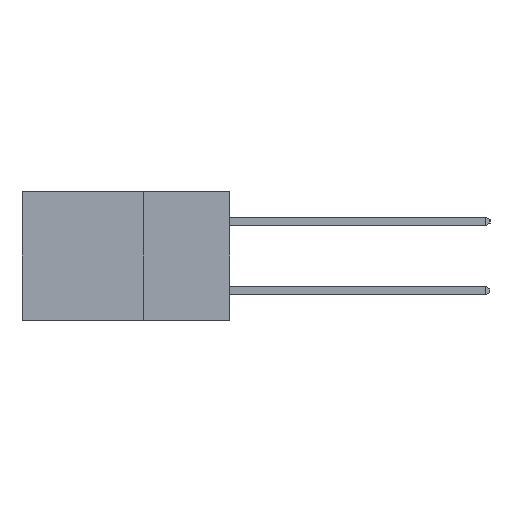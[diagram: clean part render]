
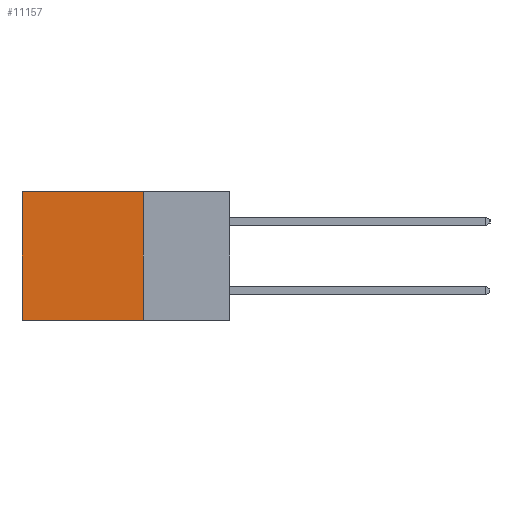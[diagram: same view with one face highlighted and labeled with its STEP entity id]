
A CAD part, left-side view. The second image highlights one B-rep face of the part: STEP entity #11157.
In plain terms, the highlighted planar face has unit normal (-1, 0, 0).
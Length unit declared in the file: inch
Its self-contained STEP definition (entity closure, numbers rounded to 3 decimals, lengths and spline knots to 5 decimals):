
#114 = CARTESIAN_POINT ( 'NONE',  ( 0.298, 0.6, 0. ) ) ;
#216 = VECTOR ( 'NONE', #2900, 39.37008 ) ;
#567 = VECTOR ( 'NONE', #4350, 39.37008 ) ;
#844 = ORIENTED_EDGE ( 'NONE', *, *, #13012, .T. ) ;
#1323 = LINE ( 'NONE', #11193, #3573 ) ;
#1818 = DIRECTION ( 'NONE',  ( 0., 0., -1. ) ) ;
#1837 = DIRECTION ( 'NONE',  ( 1., 0., 0. ) ) ;
#1908 = PLANE ( 'NONE',  #3236 ) ;
#1910 = ORIENTED_EDGE ( 'NONE', *, *, #11044, .T. ) ;
#1998 = VERTEX_POINT ( 'NONE', #114 ) ;
#2043 = CARTESIAN_POINT ( 'NONE',  ( 0.298, 0.25, 0. ) ) ;
#2697 = EDGE_LOOP ( 'NONE', ( #844, #6848, #4448, #1910 ) ) ;
#2900 = DIRECTION ( 'NONE',  ( 0., 1., 0. ) ) ;
#2950 = CARTESIAN_POINT ( 'NONE',  ( 0.298, 0.25, 0. ) ) ;
#3070 = CARTESIAN_POINT ( 'NONE',  ( 0.298, 0.6, 0. ) ) ;
#3236 = AXIS2_PLACEMENT_3D ( 'NONE', #2043, #1837, #1818 ) ;
#3573 = VECTOR ( 'NONE', #6476, 39.37008 ) ;
#4350 = DIRECTION ( 'NONE',  ( 0., 0., -1. ) ) ;
#4448 = ORIENTED_EDGE ( 'NONE', *, *, #4717, .F. ) ;
#4514 = VERTEX_POINT ( 'NONE', #5156 ) ;
#4717 = EDGE_CURVE ( 'NONE', #9483, #9726, #15726, .T. ) ;
#5156 = CARTESIAN_POINT ( 'NONE',  ( 0.298, 0.6, -0.37 ) ) ;
#6476 = DIRECTION ( 'NONE',  ( 0., 1., 0. ) ) ;
#6848 = ORIENTED_EDGE ( 'NONE', *, *, #14731, .F. ) ;
#8232 = FACE_OUTER_BOUND ( 'NONE', #2697, .T. ) ;
#9206 = DIRECTION ( 'NONE',  ( 0., 0., -1. ) ) ;
#9415 = VECTOR ( 'NONE', #9206, 39.37008 ) ;
#9483 = VERTEX_POINT ( 'NONE', #15232 ) ;
#9726 = VERTEX_POINT ( 'NONE', #13757 ) ;
#10098 = LINE ( 'NONE', #2950, #216 ) ;
#10411 = LINE ( 'NONE', #3070, #567 ) ;
#11044 = EDGE_CURVE ( 'NONE', #9483, #1998, #10098, .T. ) ;
#11157 = ADVANCED_FACE ( 'NONE', ( #8232 ), #1908, .F. ) ;
#11193 = CARTESIAN_POINT ( 'NONE',  ( 0.298, 0.25, -0.37 ) ) ;
#13012 = EDGE_CURVE ( 'NONE', #1998, #4514, #10411, .T. ) ;
#13757 = CARTESIAN_POINT ( 'NONE',  ( 0.298, 0.25, -0.37 ) ) ;
#14731 = EDGE_CURVE ( 'NONE', #9726, #4514, #1323, .T. ) ;
#14793 = CARTESIAN_POINT ( 'NONE',  ( 0.298, 0.25, 0. ) ) ;
#15232 = CARTESIAN_POINT ( 'NONE',  ( 0.298, 0.25, 0. ) ) ;
#15726 = LINE ( 'NONE', #14793, #9415 ) ;
